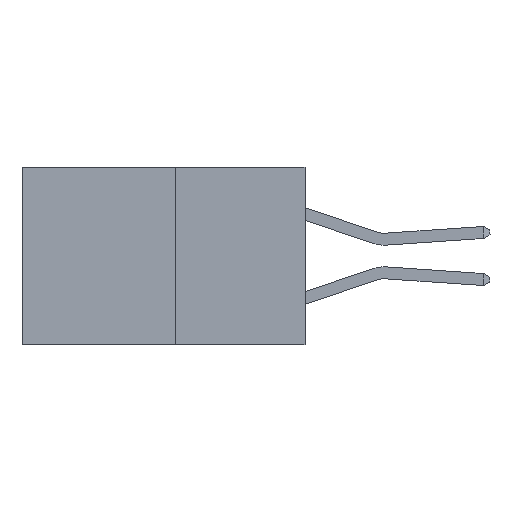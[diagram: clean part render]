
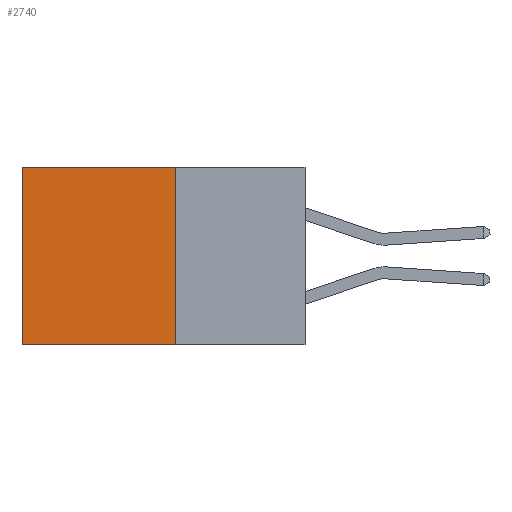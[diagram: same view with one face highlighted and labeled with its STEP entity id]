
A CAD part, left-side view. The second image highlights one B-rep face of the part: STEP entity #2740.
In plain terms, the highlighted planar face has unit normal (-1, 0, 0).
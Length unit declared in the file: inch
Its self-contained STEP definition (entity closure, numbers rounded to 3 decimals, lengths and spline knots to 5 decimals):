
#90 = DIRECTION ( 'NONE',  ( 0., 0., -1. ) ) ;
#312 = CARTESIAN_POINT ( 'NONE',  ( 0.277, 0.27, 0. ) ) ;
#472 = ORIENTED_EDGE ( 'NONE', *, *, #5558, .T. ) ;
#501 = CARTESIAN_POINT ( 'NONE',  ( 0.277, 0.59, -0.37 ) ) ;
#797 = EDGE_CURVE ( 'NONE', #6689, #2949, #4907, .T. ) ;
#854 = VECTOR ( 'NONE', #7550, 39.37008 ) ;
#1117 = LINE ( 'NONE', #8440, #8721 ) ;
#1761 = VERTEX_POINT ( 'NONE', #312 ) ;
#2118 = DIRECTION ( 'NONE',  ( 0., 1., 0. ) ) ;
#2168 = CARTESIAN_POINT ( 'NONE',  ( 0.277, 0.27, 0. ) ) ;
#2607 = ORIENTED_EDGE ( 'NONE', *, *, #797, .F. ) ;
#2614 = VERTEX_POINT ( 'NONE', #3357 ) ;
#2740 = ADVANCED_FACE ( 'NONE', ( #2919 ), #8802, .F. ) ;
#2919 = FACE_OUTER_BOUND ( 'NONE', #2988, .T. ) ;
#2949 = VERTEX_POINT ( 'NONE', #8781 ) ;
#2988 = EDGE_LOOP ( 'NONE', ( #472, #2607, #4550, #6473 ) ) ;
#3215 = LINE ( 'NONE', #501, #6855 ) ;
#3357 = CARTESIAN_POINT ( 'NONE',  ( 0.277, 0.59, 0. ) ) ;
#4350 = AXIS2_PLACEMENT_3D ( 'NONE', #8768, #8742, #8696 ) ;
#4550 = ORIENTED_EDGE ( 'NONE', *, *, #6931, .F. ) ;
#4745 = EDGE_CURVE ( 'NONE', #1761, #2614, #6981, .T. ) ;
#4907 = LINE ( 'NONE', #6312, #854 ) ;
#4992 = VECTOR ( 'NONE', #2118, 39.37008 ) ;
#5414 = CARTESIAN_POINT ( 'NONE',  ( 0.277, 0.27, -0.37 ) ) ;
#5558 = EDGE_CURVE ( 'NONE', #2614, #2949, #3215, .T. ) ;
#5598 = DIRECTION ( 'NONE',  ( 0., 0., -1. ) ) ;
#6312 = CARTESIAN_POINT ( 'NONE',  ( 0.277, 0.27, -0.37 ) ) ;
#6473 = ORIENTED_EDGE ( 'NONE', *, *, #4745, .T. ) ;
#6689 = VERTEX_POINT ( 'NONE', #5414 ) ;
#6855 = VECTOR ( 'NONE', #90, 39.37008 ) ;
#6931 = EDGE_CURVE ( 'NONE', #1761, #6689, #1117, .T. ) ;
#6981 = LINE ( 'NONE', #2168, #4992 ) ;
#7550 = DIRECTION ( 'NONE',  ( 0., 1., 0. ) ) ;
#8440 = CARTESIAN_POINT ( 'NONE',  ( 0.277, 0.27, -0.37 ) ) ;
#8696 = DIRECTION ( 'NONE',  ( 0., 0., -1. ) ) ;
#8721 = VECTOR ( 'NONE', #5598, 39.37008 ) ;
#8742 = DIRECTION ( 'NONE',  ( 1., 0., 0. ) ) ;
#8768 = CARTESIAN_POINT ( 'NONE',  ( 0.277, 0.27, -0.37 ) ) ;
#8781 = CARTESIAN_POINT ( 'NONE',  ( 0.277, 0.59, -0.37 ) ) ;
#8802 = PLANE ( 'NONE',  #4350 ) ;
